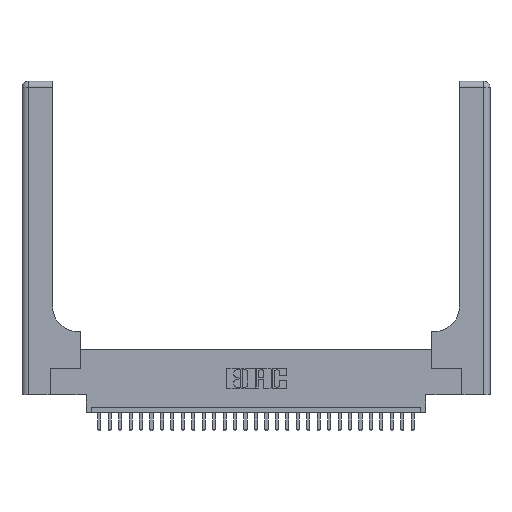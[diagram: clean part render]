
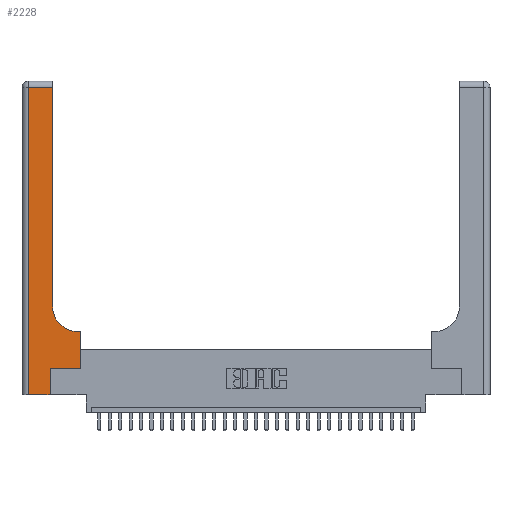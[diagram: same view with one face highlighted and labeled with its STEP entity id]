
A CAD part, top view. The second image highlights one B-rep face of the part: STEP entity #2228.
In plain terms, the highlighted planar face has unit normal (0, 0, 1).
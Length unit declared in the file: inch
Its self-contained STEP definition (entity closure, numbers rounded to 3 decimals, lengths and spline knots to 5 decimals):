
#6 = CARTESIAN_POINT ( 'NONE',  ( 0., 0., 0.37 ) ) ;
#278 = VERTEX_POINT ( 'NONE', #29407 ) ;
#394 = EDGE_CURVE ( 'NONE', #18861, #4001, #21214, .T. ) ;
#536 = CARTESIAN_POINT ( 'NONE',  ( 0.5415, 0.6, 0.37 ) ) ;
#763 = VERTEX_POINT ( 'NONE', #13447 ) ;
#927 = DIRECTION ( 'NONE',  ( -1., 0., 0. ) ) ;
#1297 = CARTESIAN_POINT ( 'NONE',  ( 0.5415, 0.85, 0.37 ) ) ;
#1444 = VECTOR ( 'NONE', #927, 39.37008 ) ;
#1493 = DIRECTION ( 'NONE',  ( 0., 0., -1. ) ) ;
#1576 = EDGE_CURVE ( 'NONE', #21021, #3760, #3272, .T. ) ;
#2228 = ADVANCED_FACE ( 'NONE', ( #8725 ), #24064, .F. ) ;
#2254 = EDGE_LOOP ( 'NONE', ( #10185, #5064, #20548, #21113, #5410, #26881, #5324, #22286, #3738 ) ) ;
#2410 = EDGE_CURVE ( 'NONE', #18331, #278, #27353, .T. ) ;
#3272 = LINE ( 'NONE', #22130, #1444 ) ;
#3399 = AXIS2_PLACEMENT_3D ( 'NONE', #10128, #19350, #10541 ) ;
#3738 = ORIENTED_EDGE ( 'NONE', *, *, #25382, .T. ) ;
#3760 = VERTEX_POINT ( 'NONE', #536 ) ;
#4001 = VERTEX_POINT ( 'NONE', #22800 ) ;
#4346 = DIRECTION ( 'NONE',  ( 0., -1., 0. ) ) ;
#4893 = CARTESIAN_POINT ( 'NONE',  ( 0.06, 2.94, 0.37 ) ) ;
#4934 = DIRECTION ( 'NONE',  ( 0., 1., 0. ) ) ;
#5064 = ORIENTED_EDGE ( 'NONE', *, *, #16707, .T. ) ;
#5324 = ORIENTED_EDGE ( 'NONE', *, *, #23565, .T. ) ;
#5410 = ORIENTED_EDGE ( 'NONE', *, *, #394, .T. ) ;
#6186 = VERTEX_POINT ( 'NONE', #18199 ) ;
#7918 = CARTESIAN_POINT ( 'NONE',  ( 0.5585, 0.25, 0.37 ) ) ;
#8111 = DIRECTION ( 'NONE',  ( 0., 1., 0. ) ) ;
#8725 = FACE_OUTER_BOUND ( 'NONE', #2254, .T. ) ;
#9198 = DIRECTION ( 'NONE',  ( 0., 1., 0. ) ) ;
#10128 = CARTESIAN_POINT ( 'NONE',  ( 0., 3., 0.37 ) ) ;
#10185 = ORIENTED_EDGE ( 'NONE', *, *, #14464, .T. ) ;
#10541 = DIRECTION ( 'NONE',  ( -1., 0., 0. ) ) ;
#10958 = DIRECTION ( 'NONE',  ( -1., 0., 0. ) ) ;
#10967 = CARTESIAN_POINT ( 'NONE',  ( 0.2915, 2.94, 0.37 ) ) ;
#13348 = VECTOR ( 'NONE', #8111, 39.37008 ) ;
#13403 = CARTESIAN_POINT ( 'NONE',  ( 0., 2.94, 0.37 ) ) ;
#13447 = CARTESIAN_POINT ( 'NONE',  ( 0.5585, 0.25, 0.37 ) ) ;
#13767 = CARTESIAN_POINT ( 'NONE',  ( 0.5585, 0.6, 0.37 ) ) ;
#14464 = EDGE_CURVE ( 'NONE', #6186, #23714, #18266, .T. ) ;
#15457 = CIRCLE ( 'NONE', #30217, 0.25 ) ;
#15666 = VECTOR ( 'NONE', #4346, 39.37008 ) ;
#15923 = CARTESIAN_POINT ( 'NONE',  ( 0.269, 0., 0.37 ) ) ;
#16151 = LINE ( 'NONE', #6, #25638 ) ;
#16707 = EDGE_CURVE ( 'NONE', #23714, #18331, #30151, .T. ) ;
#17571 = DIRECTION ( 'NONE',  ( 1., 0., 0. ) ) ;
#18199 = CARTESIAN_POINT ( 'NONE',  ( 0.2915, 0.85, 0.37 ) ) ;
#18266 = LINE ( 'NONE', #28238, #21181 ) ;
#18331 = VERTEX_POINT ( 'NONE', #4893 ) ;
#18861 = VERTEX_POINT ( 'NONE', #27175 ) ;
#18941 = DIRECTION ( 'NONE',  ( 1., 0., 0. ) ) ;
#19350 = DIRECTION ( 'NONE',  ( 0., 0., -1. ) ) ;
#19527 = LINE ( 'NONE', #7918, #13348 ) ;
#20548 = ORIENTED_EDGE ( 'NONE', *, *, #2410, .T. ) ;
#20986 = EDGE_CURVE ( 'NONE', #4001, #763, #28102, .T. ) ;
#21021 = VERTEX_POINT ( 'NONE', #13767 ) ;
#21113 = ORIENTED_EDGE ( 'NONE', *, *, #26014, .T. ) ;
#21181 = VECTOR ( 'NONE', #4934, 39.37008 ) ;
#21214 = LINE ( 'NONE', #15923, #27830 ) ;
#22130 = CARTESIAN_POINT ( 'NONE',  ( 0.2915, 0.6, 0.37 ) ) ;
#22224 = CARTESIAN_POINT ( 'NONE',  ( 0.06, 3., 0.37 ) ) ;
#22286 = ORIENTED_EDGE ( 'NONE', *, *, #1576, .T. ) ;
#22800 = CARTESIAN_POINT ( 'NONE',  ( 0.269, 0.25, 0.37 ) ) ;
#23565 = EDGE_CURVE ( 'NONE', #763, #21021, #19527, .T. ) ;
#23714 = VERTEX_POINT ( 'NONE', #10967 ) ;
#24064 = PLANE ( 'NONE',  #3399 ) ;
#24265 = VECTOR ( 'NONE', #10958, 39.37008 ) ;
#25382 = EDGE_CURVE ( 'NONE', #3760, #6186, #15457, .T. ) ;
#25638 = VECTOR ( 'NONE', #18941, 39.37008 ) ;
#26014 = EDGE_CURVE ( 'NONE', #278, #18861, #16151, .T. ) ;
#26881 = ORIENTED_EDGE ( 'NONE', *, *, #20986, .T. ) ;
#27175 = CARTESIAN_POINT ( 'NONE',  ( 0.269, 0., 0.37 ) ) ;
#27353 = LINE ( 'NONE', #22224, #15666 ) ;
#27359 = VECTOR ( 'NONE', #27448, 39.37008 ) ;
#27448 = DIRECTION ( 'NONE',  ( 1., 0., 0. ) ) ;
#27830 = VECTOR ( 'NONE', #9198, 39.37008 ) ;
#28102 = LINE ( 'NONE', #30215, #27359 ) ;
#28238 = CARTESIAN_POINT ( 'NONE',  ( 0.2915, 3., 0.37 ) ) ;
#29407 = CARTESIAN_POINT ( 'NONE',  ( 0.06, 0., 0.37 ) ) ;
#30151 = LINE ( 'NONE', #13403, #24265 ) ;
#30215 = CARTESIAN_POINT ( 'NONE',  ( 0.269, 0.25, 0.37 ) ) ;
#30217 = AXIS2_PLACEMENT_3D ( 'NONE', #1297, #1493, #17571 ) ;
